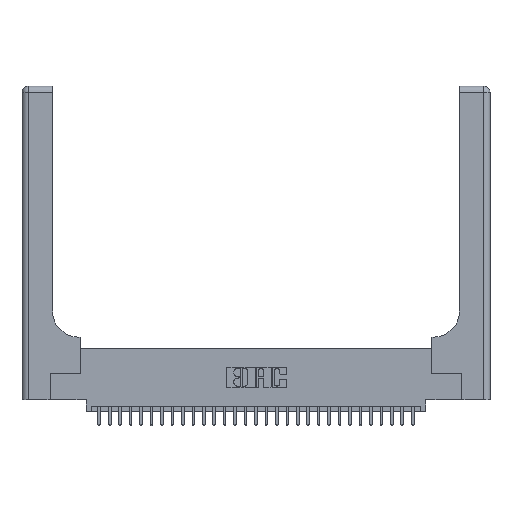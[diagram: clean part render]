
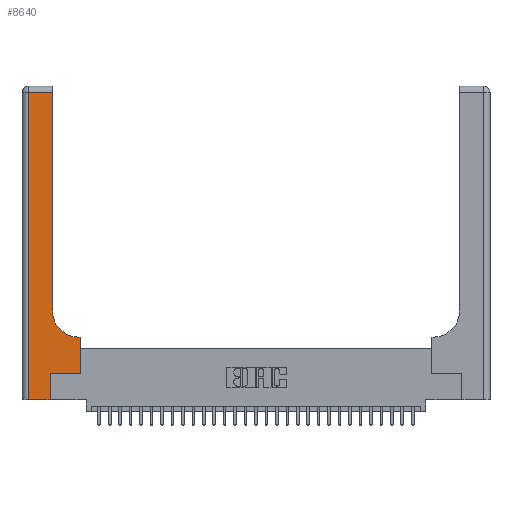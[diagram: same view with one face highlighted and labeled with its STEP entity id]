
A CAD part, top view. The second image highlights one B-rep face of the part: STEP entity #8640.
In plain terms, the highlighted planar face has unit normal (0, 0, 1).
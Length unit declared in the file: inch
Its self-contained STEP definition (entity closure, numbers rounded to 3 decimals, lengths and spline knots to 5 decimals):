
#89 = CARTESIAN_POINT ( 'NONE',  ( 0.5415, 0.6, 0.37 ) ) ;
#857 = CARTESIAN_POINT ( 'NONE',  ( 0.2915, 0.6, 0.37 ) ) ;
#1170 = VERTEX_POINT ( 'NONE', #16106 ) ;
#1550 = DIRECTION ( 'NONE',  ( 0., 1., 0. ) ) ;
#1608 = CARTESIAN_POINT ( 'NONE',  ( 0.5585, 0.25, 0.37 ) ) ;
#2170 = LINE ( 'NONE', #10313, #7098 ) ;
#3143 = LINE ( 'NONE', #20769, #28001 ) ;
#3445 = DIRECTION ( 'NONE',  ( 0., 1., 0. ) ) ;
#4084 = CARTESIAN_POINT ( 'NONE',  ( 0.06, 2.94, 0.37 ) ) ;
#4488 = CARTESIAN_POINT ( 'NONE',  ( 0.2915, 0.85, 0.37 ) ) ;
#4650 = EDGE_CURVE ( 'NONE', #8135, #19831, #18972, .T. ) ;
#5117 = VECTOR ( 'NONE', #22424, 39.37008 ) ;
#5568 = CARTESIAN_POINT ( 'NONE',  ( 0.06, 3., 0.37 ) ) ;
#5762 = ORIENTED_EDGE ( 'NONE', *, *, #18311, .T. ) ;
#7098 = VECTOR ( 'NONE', #21916, 39.37008 ) ;
#7246 = ORIENTED_EDGE ( 'NONE', *, *, #28712, .T. ) ;
#7462 = EDGE_CURVE ( 'NONE', #28985, #1170, #15385, .T. ) ;
#7793 = ORIENTED_EDGE ( 'NONE', *, *, #30935, .T. ) ;
#8135 = VERTEX_POINT ( 'NONE', #13359 ) ;
#8640 = ADVANCED_FACE ( 'NONE', ( #14928 ), #24104, .F. ) ;
#9484 = AXIS2_PLACEMENT_3D ( 'NONE', #31006, #9717, #18838 ) ;
#9717 = DIRECTION ( 'NONE',  ( 0., 0., -1. ) ) ;
#10313 = CARTESIAN_POINT ( 'NONE',  ( 0., 0., 0.37 ) ) ;
#10332 = VERTEX_POINT ( 'NONE', #4488 ) ;
#11094 = EDGE_LOOP ( 'NONE', ( #21978, #26758, #7246, #5762, #20841, #22735, #12325, #26442, #7793 ) ) ;
#11150 = CARTESIAN_POINT ( 'NONE',  ( 0.269, 0., 0.37 ) ) ;
#11419 = VECTOR ( 'NONE', #22450, 39.37008 ) ;
#12325 = ORIENTED_EDGE ( 'NONE', *, *, #4650, .T. ) ;
#12489 = CARTESIAN_POINT ( 'NONE',  ( 0.269, 0.25, 0.37 ) ) ;
#13359 = CARTESIAN_POINT ( 'NONE',  ( 0.5585, 0.25, 0.37 ) ) ;
#14037 = EDGE_CURVE ( 'NONE', #1170, #8135, #29168, .T. ) ;
#14294 = CARTESIAN_POINT ( 'NONE',  ( 0.5585, 0.6, 0.37 ) ) ;
#14928 = FACE_OUTER_BOUND ( 'NONE', #11094, .T. ) ;
#15012 = DIRECTION ( 'NONE',  ( 1., 0., 0. ) ) ;
#15385 = LINE ( 'NONE', #15813, #28872 ) ;
#15813 = CARTESIAN_POINT ( 'NONE',  ( 0.269, 0., 0.37 ) ) ;
#16106 = CARTESIAN_POINT ( 'NONE',  ( 0.269, 0.25, 0.37 ) ) ;
#16207 = EDGE_CURVE ( 'NONE', #19831, #20032, #19285, .T. ) ;
#16655 = EDGE_CURVE ( 'NONE', #18991, #25312, #26005, .T. ) ;
#16713 = CIRCLE ( 'NONE', #24430, 0.25 ) ;
#16822 = CARTESIAN_POINT ( 'NONE',  ( 0., 2.94, 0.37 ) ) ;
#17632 = DIRECTION ( 'NONE',  ( -1., 0., 0. ) ) ;
#18311 = EDGE_CURVE ( 'NONE', #19814, #28985, #2170, .T. ) ;
#18838 = DIRECTION ( 'NONE',  ( -1., 0., 0. ) ) ;
#18972 = LINE ( 'NONE', #1608, #28720 ) ;
#18991 = VERTEX_POINT ( 'NONE', #25327 ) ;
#19285 = LINE ( 'NONE', #857, #24924 ) ;
#19736 = EDGE_CURVE ( 'NONE', #10332, #18991, #3143, .T. ) ;
#19814 = VERTEX_POINT ( 'NONE', #30833 ) ;
#19831 = VERTEX_POINT ( 'NONE', #14294 ) ;
#20032 = VERTEX_POINT ( 'NONE', #89 ) ;
#20769 = CARTESIAN_POINT ( 'NONE',  ( 0.2915, 3., 0.37 ) ) ;
#20841 = ORIENTED_EDGE ( 'NONE', *, *, #7462, .T. ) ;
#21916 = DIRECTION ( 'NONE',  ( 1., 0., 0. ) ) ;
#21978 = ORIENTED_EDGE ( 'NONE', *, *, #19736, .T. ) ;
#22424 = DIRECTION ( 'NONE',  ( 0., -1., 0. ) ) ;
#22450 = DIRECTION ( 'NONE',  ( -1., 0., 0. ) ) ;
#22735 = ORIENTED_EDGE ( 'NONE', *, *, #14037, .T. ) ;
#22799 = VECTOR ( 'NONE', #29251, 39.37008 ) ;
#24104 = PLANE ( 'NONE',  #9484 ) ;
#24430 = AXIS2_PLACEMENT_3D ( 'NONE', #29461, #29360, #15012 ) ;
#24924 = VECTOR ( 'NONE', #17632, 39.37008 ) ;
#25312 = VERTEX_POINT ( 'NONE', #4084 ) ;
#25327 = CARTESIAN_POINT ( 'NONE',  ( 0.2915, 2.94, 0.37 ) ) ;
#25867 = LINE ( 'NONE', #5568, #5117 ) ;
#26005 = LINE ( 'NONE', #16822, #11419 ) ;
#26442 = ORIENTED_EDGE ( 'NONE', *, *, #16207, .T. ) ;
#26758 = ORIENTED_EDGE ( 'NONE', *, *, #16655, .T. ) ;
#28001 = VECTOR ( 'NONE', #30518, 39.37008 ) ;
#28712 = EDGE_CURVE ( 'NONE', #25312, #19814, #25867, .T. ) ;
#28720 = VECTOR ( 'NONE', #3445, 39.37008 ) ;
#28872 = VECTOR ( 'NONE', #1550, 39.37008 ) ;
#28985 = VERTEX_POINT ( 'NONE', #11150 ) ;
#29168 = LINE ( 'NONE', #12489, #22799 ) ;
#29251 = DIRECTION ( 'NONE',  ( 1., 0., 0. ) ) ;
#29360 = DIRECTION ( 'NONE',  ( 0., 0., -1. ) ) ;
#29461 = CARTESIAN_POINT ( 'NONE',  ( 0.5415, 0.85, 0.37 ) ) ;
#30518 = DIRECTION ( 'NONE',  ( 0., 1., 0. ) ) ;
#30833 = CARTESIAN_POINT ( 'NONE',  ( 0.06, 0., 0.37 ) ) ;
#30935 = EDGE_CURVE ( 'NONE', #20032, #10332, #16713, .T. ) ;
#31006 = CARTESIAN_POINT ( 'NONE',  ( 0., 3., 0.37 ) ) ;
